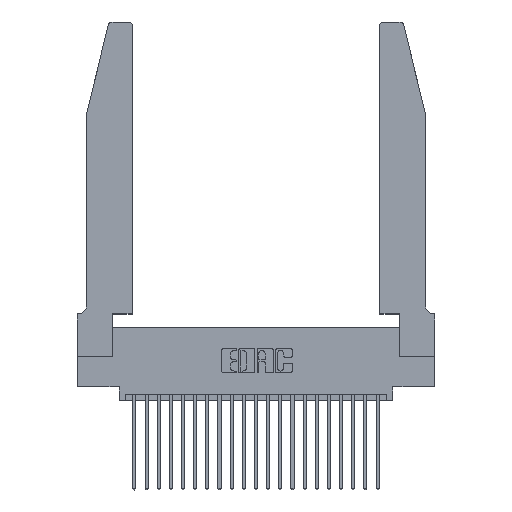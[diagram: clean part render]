
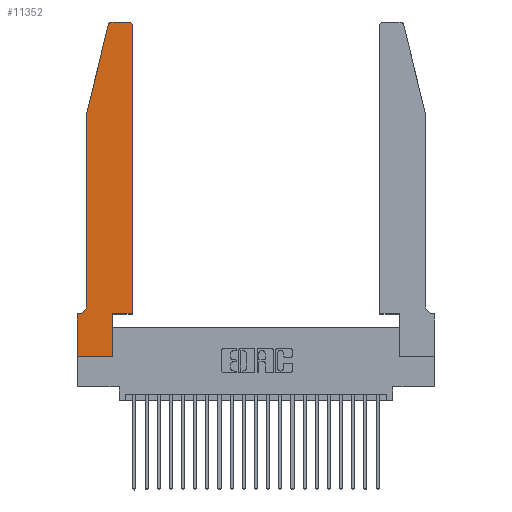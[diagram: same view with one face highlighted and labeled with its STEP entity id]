
A CAD part, top view. The second image highlights one B-rep face of the part: STEP entity #11352.
In plain terms, the highlighted planar face has unit normal (0, 0, 1).
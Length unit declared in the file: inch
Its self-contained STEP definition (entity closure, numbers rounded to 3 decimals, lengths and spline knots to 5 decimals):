
#256 = LINE ( 'NONE', #6268, #10550 ) ;
#359 = CARTESIAN_POINT ( 'NONE',  ( 0.4205, 2.75, 0.37 ) ) ;
#754 = DIRECTION ( 'NONE',  ( 0., 0., -1. ) ) ;
#1379 = DIRECTION ( 'NONE',  ( 1., 0., 0. ) ) ;
#1643 = DIRECTION ( 'NONE',  ( 0., 0., 1. ) ) ;
#1704 = EDGE_CURVE ( 'NONE', #18013, #12190, #17758, .T. ) ;
#1800 = DIRECTION ( 'NONE',  ( 1., 0., 0. ) ) ;
#2360 = AXIS2_PLACEMENT_3D ( 'NONE', #2494, #2413, #22994 ) ;
#2413 = DIRECTION ( 'NONE',  ( 0., 0., 1. ) ) ;
#2494 = CARTESIAN_POINT ( 'NONE',  ( 0., 0.35, 0.37 ) ) ;
#3540 = CARTESIAN_POINT ( 'NONE',  ( 0.4505, 2.72, 0.37 ) ) ;
#3596 = AXIS2_PLACEMENT_3D ( 'NONE', #15715, #754, #10180 ) ;
#3621 = EDGE_CURVE ( 'NONE', #7861, #8747, #8623, .T. ) ;
#4001 = CARTESIAN_POINT ( 'NONE',  ( 0.4505, 0.35, 0.37 ) ) ;
#4106 = AXIS2_PLACEMENT_3D ( 'NONE', #18127, #14376, #1379 ) ;
#4136 = LINE ( 'NONE', #22926, #23448 ) ;
#4323 = VECTOR ( 'NONE', #15700, 39.37008 ) ;
#4622 = ORIENTED_EDGE ( 'NONE', *, *, #18799, .T. ) ;
#4703 = ORIENTED_EDGE ( 'NONE', *, *, #20525, .T. ) ;
#4933 = CARTESIAN_POINT ( 'NONE',  ( 0.2865, 0.35, 0.37 ) ) ;
#5761 = DIRECTION ( 'NONE',  ( -1., 0., 0. ) ) ;
#6268 = CARTESIAN_POINT ( 'NONE',  ( 0.0755, 2., 0.37 ) ) ;
#6679 = VERTEX_POINT ( 'NONE', #21942 ) ;
#6704 = VERTEX_POINT ( 'NONE', #9120 ) ;
#6879 = ORIENTED_EDGE ( 'NONE', *, *, #15150, .T. ) ;
#7360 = CARTESIAN_POINT ( 'NONE',  ( 0.25487, 2.72718, 0.37 ) ) ;
#7417 = VERTEX_POINT ( 'NONE', #20992 ) ;
#7861 = VERTEX_POINT ( 'NONE', #3540 ) ;
#8345 = CARTESIAN_POINT ( 'NONE',  ( 0.0755, 0.35, 0.37 ) ) ;
#8623 = CIRCLE ( 'NONE', #20193, 0.03 ) ;
#8747 = VERTEX_POINT ( 'NONE', #359 ) ;
#8789 = VECTOR ( 'NONE', #23395, 39.37008 ) ;
#8965 = VERTEX_POINT ( 'NONE', #13043 ) ;
#9120 = CARTESIAN_POINT ( 'NONE',  ( 0.0755, 2., 0.37 ) ) ;
#9362 = VECTOR ( 'NONE', #13372, 39.37008 ) ;
#10019 = EDGE_CURVE ( 'NONE', #6704, #6679, #256, .T. ) ;
#10180 = DIRECTION ( 'NONE',  ( -1., 0., 0. ) ) ;
#10405 = EDGE_CURVE ( 'NONE', #8965, #7417, #15195, .T. ) ;
#10506 = CIRCLE ( 'NONE', #3596, 0.07 ) ;
#10550 = VECTOR ( 'NONE', #15590, 39.37008 ) ;
#10688 = LINE ( 'NONE', #22607, #19418 ) ;
#10708 = DIRECTION ( 'NONE',  ( 0., 1., 0. ) ) ;
#11352 = ADVANCED_FACE ( 'NONE', ( #17205 ), #15241, .T. ) ;
#11478 = VERTEX_POINT ( 'NONE', #13852 ) ;
#11924 = LINE ( 'NONE', #21329, #19211 ) ;
#12184 = LINE ( 'NONE', #20000, #19764 ) ;
#12190 = VERTEX_POINT ( 'NONE', #18550 ) ;
#12254 = VERTEX_POINT ( 'NONE', #7360 ) ;
#12280 = ORIENTED_EDGE ( 'NONE', *, *, #10405, .T. ) ;
#12798 = EDGE_CURVE ( 'NONE', #11478, #7861, #12184, .T. ) ;
#13043 = CARTESIAN_POINT ( 'NONE',  ( 0.2865, 0., 0.37 ) ) ;
#13372 = DIRECTION ( 'NONE',  ( 1., 0., 0. ) ) ;
#13447 = DIRECTION ( 'NONE',  ( -0.239, -0.971, 0. ) ) ;
#13852 = CARTESIAN_POINT ( 'NONE',  ( 0.4505, 0.35, 0.37 ) ) ;
#13896 = CIRCLE ( 'NONE', #4106, 0.03 ) ;
#14012 = EDGE_CURVE ( 'NONE', #20272, #12254, #13896, .T. ) ;
#14281 = EDGE_CURVE ( 'NONE', #8747, #20272, #10688, .T. ) ;
#14376 = DIRECTION ( 'NONE',  ( 0., 0., 1. ) ) ;
#15037 = ORIENTED_EDGE ( 'NONE', *, *, #15116, .T. ) ;
#15116 = EDGE_CURVE ( 'NONE', #12190, #23482, #11924, .T. ) ;
#15150 = EDGE_CURVE ( 'NONE', #23482, #8965, #20404, .T. ) ;
#15195 = LINE ( 'NONE', #4933, #8789 ) ;
#15241 = PLANE ( 'NONE',  #2360 ) ;
#15555 = CARTESIAN_POINT ( 'NONE',  ( 0.0055, 0.35, 0.37 ) ) ;
#15590 = DIRECTION ( 'NONE',  ( 0., -1., 0. ) ) ;
#15700 = DIRECTION ( 'NONE',  ( 1., 0., 0. ) ) ;
#15715 = CARTESIAN_POINT ( 'NONE',  ( 0.0055, 0.42, 0.37 ) ) ;
#15842 = DIRECTION ( 'NONE',  ( -1., 0., 0. ) ) ;
#16917 = ORIENTED_EDGE ( 'NONE', *, *, #14281, .T. ) ;
#17106 = EDGE_LOOP ( 'NONE', ( #16917, #18242, #4622, #21569, #22578, #19573, #15037, #6879, #12280, #4703, #23640, #22028 ) ) ;
#17205 = FACE_OUTER_BOUND ( 'NONE', #17106, .T. ) ;
#17410 = CARTESIAN_POINT ( 'NONE',  ( 0., 0., 0.37 ) ) ;
#17758 = LINE ( 'NONE', #8345, #18644 ) ;
#17837 = LINE ( 'NONE', #4001, #9362 ) ;
#18013 = VERTEX_POINT ( 'NONE', #15555 ) ;
#18127 = CARTESIAN_POINT ( 'NONE',  ( 0.284, 2.72, 0.37 ) ) ;
#18148 = CARTESIAN_POINT ( 'NONE',  ( 0.284, 2.75, 0.37 ) ) ;
#18242 = ORIENTED_EDGE ( 'NONE', *, *, #14012, .T. ) ;
#18550 = CARTESIAN_POINT ( 'NONE',  ( 0., 0.35, 0.37 ) ) ;
#18644 = VECTOR ( 'NONE', #15842, 39.37008 ) ;
#18799 = EDGE_CURVE ( 'NONE', #12254, #6704, #4136, .T. ) ;
#19191 = DIRECTION ( 'NONE',  ( 0., -1., 0. ) ) ;
#19211 = VECTOR ( 'NONE', #19191, 39.37008 ) ;
#19418 = VECTOR ( 'NONE', #5761, 39.37008 ) ;
#19480 = CARTESIAN_POINT ( 'NONE',  ( 0., 0., 0.37 ) ) ;
#19573 = ORIENTED_EDGE ( 'NONE', *, *, #1704, .T. ) ;
#19764 = VECTOR ( 'NONE', #10708, 39.37008 ) ;
#20000 = CARTESIAN_POINT ( 'NONE',  ( 0.4505, 0.35, 0.37 ) ) ;
#20193 = AXIS2_PLACEMENT_3D ( 'NONE', #21986, #1643, #1800 ) ;
#20272 = VERTEX_POINT ( 'NONE', #18148 ) ;
#20404 = LINE ( 'NONE', #17410, #4323 ) ;
#20525 = EDGE_CURVE ( 'NONE', #7417, #11478, #17837, .T. ) ;
#20992 = CARTESIAN_POINT ( 'NONE',  ( 0.2865, 0.35, 0.37 ) ) ;
#21269 = EDGE_CURVE ( 'NONE', #6679, #18013, #10506, .T. ) ;
#21329 = CARTESIAN_POINT ( 'NONE',  ( 0., 0., 0.37 ) ) ;
#21569 = ORIENTED_EDGE ( 'NONE', *, *, #10019, .T. ) ;
#21942 = CARTESIAN_POINT ( 'NONE',  ( 0.0755, 0.42, 0.37 ) ) ;
#21986 = CARTESIAN_POINT ( 'NONE',  ( 0.4205, 2.72, 0.37 ) ) ;
#22028 = ORIENTED_EDGE ( 'NONE', *, *, #3621, .T. ) ;
#22578 = ORIENTED_EDGE ( 'NONE', *, *, #21269, .T. ) ;
#22607 = CARTESIAN_POINT ( 'NONE',  ( 0.2605, 2.75, 0.37 ) ) ;
#22926 = CARTESIAN_POINT ( 'NONE',  ( 0.0755, 2., 0.37 ) ) ;
#22994 = DIRECTION ( 'NONE',  ( 1., 0., 0. ) ) ;
#23395 = DIRECTION ( 'NONE',  ( 0., 1., 0. ) ) ;
#23448 = VECTOR ( 'NONE', #13447, 39.37008 ) ;
#23482 = VERTEX_POINT ( 'NONE', #19480 ) ;
#23640 = ORIENTED_EDGE ( 'NONE', *, *, #12798, .T. ) ;
